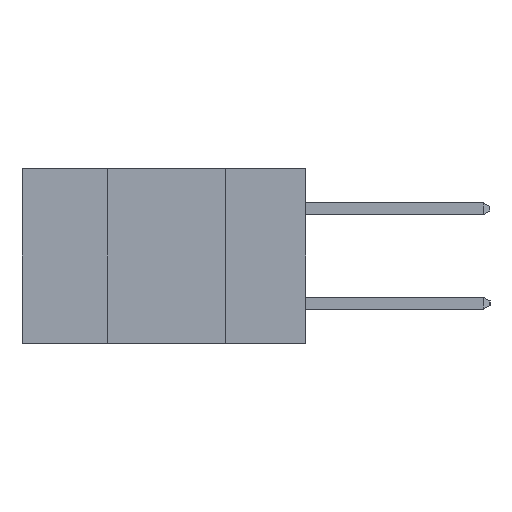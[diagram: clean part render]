
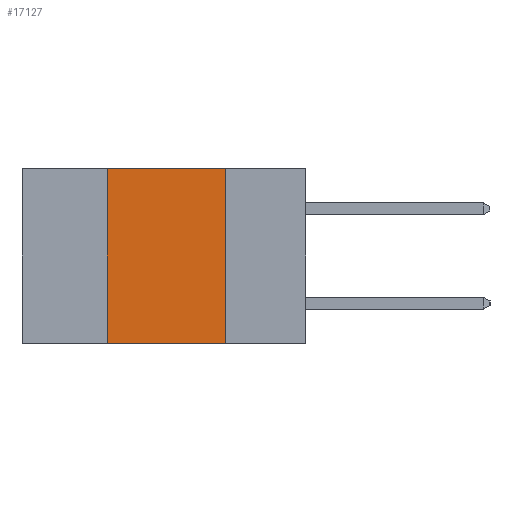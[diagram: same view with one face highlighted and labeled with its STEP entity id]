
A CAD part, left-side view. The second image highlights one B-rep face of the part: STEP entity #17127.
In plain terms, the highlighted planar face has unit normal (-1, 0, 0).
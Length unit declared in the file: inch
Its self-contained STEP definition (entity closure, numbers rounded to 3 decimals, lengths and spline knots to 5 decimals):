
#138 = VERTEX_POINT ( 'NONE', #6591 ) ;
#1189 = ORIENTED_EDGE ( 'NONE', *, *, #3747, .T. ) ;
#1191 = LINE ( 'NONE', #9660, #11561 ) ;
#1637 = ORIENTED_EDGE ( 'NONE', *, *, #6148, .F. ) ;
#2886 = DIRECTION ( 'NONE',  ( 0., 0., -1. ) ) ;
#3426 = CARTESIAN_POINT ( 'NONE',  ( 0., 0.42, -0.37 ) ) ;
#3441 = VECTOR ( 'NONE', #15942, 39.37008 ) ;
#3708 = CARTESIAN_POINT ( 'NONE',  ( 0., 0.17, -0.37 ) ) ;
#3745 = ORIENTED_EDGE ( 'NONE', *, *, #4324, .F. ) ;
#3747 = EDGE_CURVE ( 'NONE', #6381, #13728, #10519, .T. ) ;
#4324 = EDGE_CURVE ( 'NONE', #5621, #138, #1191, .T. ) ;
#5263 = EDGE_LOOP ( 'NONE', ( #5345, #3745, #1637, #1189 ) ) ;
#5345 = ORIENTED_EDGE ( 'NONE', *, *, #14685, .F. ) ;
#5621 = VERTEX_POINT ( 'NONE', #10725 ) ;
#5966 = DIRECTION ( 'NONE',  ( 0., 0., -1. ) ) ;
#6148 = EDGE_CURVE ( 'NONE', #6381, #5621, #12945, .T. ) ;
#6381 = VERTEX_POINT ( 'NONE', #3426 ) ;
#6591 = CARTESIAN_POINT ( 'NONE',  ( 0., 0.17, 0. ) ) ;
#6750 = CARTESIAN_POINT ( 'NONE',  ( 0., 0.6, -0.37 ) ) ;
#7217 = CARTESIAN_POINT ( 'NONE',  ( 0., 0.6, 0. ) ) ;
#8511 = DIRECTION ( 'NONE',  ( 0., 0., 1. ) ) ;
#8523 = CARTESIAN_POINT ( 'NONE',  ( 0., 0.42, -0.37 ) ) ;
#9400 = FACE_OUTER_BOUND ( 'NONE', #5263, .T. ) ;
#9553 = DIRECTION ( 'NONE',  ( 0., -1., 0. ) ) ;
#9660 = CARTESIAN_POINT ( 'NONE',  ( 0., 0.6, 0. ) ) ;
#9784 = VECTOR ( 'NONE', #8511, 39.37008 ) ;
#10519 = LINE ( 'NONE', #6750, #3441 ) ;
#10725 = CARTESIAN_POINT ( 'NONE',  ( 0., 0.42, 0. ) ) ;
#11561 = VECTOR ( 'NONE', #9553, 39.37008 ) ;
#12248 = VECTOR ( 'NONE', #2886, 39.37008 ) ;
#12268 = CARTESIAN_POINT ( 'NONE',  ( 0., 0.17, -0.37 ) ) ;
#12603 = PLANE ( 'NONE',  #16615 ) ;
#12681 = LINE ( 'NONE', #12268, #12248 ) ;
#12945 = LINE ( 'NONE', #8523, #9784 ) ;
#13728 = VERTEX_POINT ( 'NONE', #3708 ) ;
#13904 = DIRECTION ( 'NONE',  ( 1., 0., 0. ) ) ;
#14685 = EDGE_CURVE ( 'NONE', #138, #13728, #12681, .T. ) ;
#15942 = DIRECTION ( 'NONE',  ( 0., -1., 0. ) ) ;
#16615 = AXIS2_PLACEMENT_3D ( 'NONE', #7217, #13904, #5966 ) ;
#17127 = ADVANCED_FACE ( 'NONE', ( #9400 ), #12603, .F. ) ;
